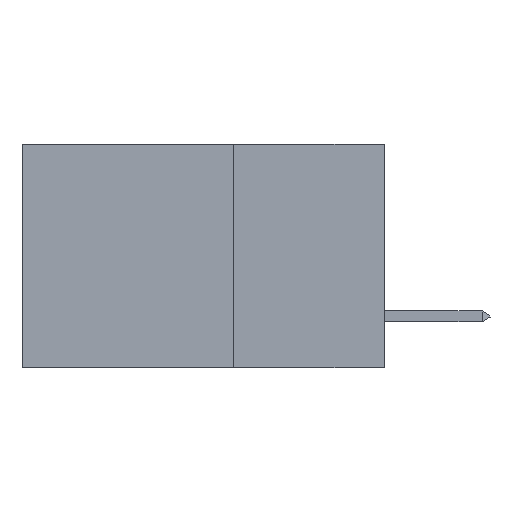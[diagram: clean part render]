
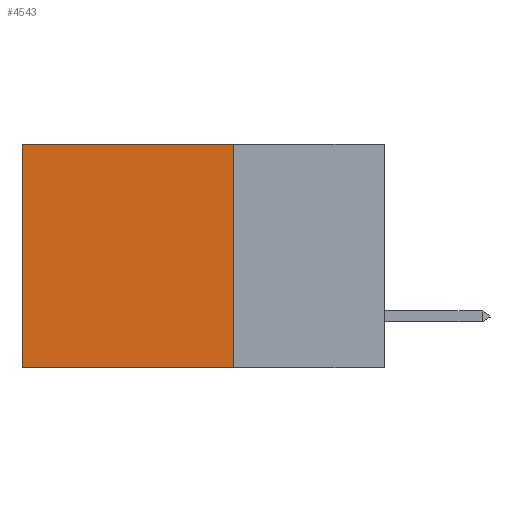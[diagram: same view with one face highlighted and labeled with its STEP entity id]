
A CAD part, left-side view. The second image highlights one B-rep face of the part: STEP entity #4543.
In plain terms, the highlighted planar face has unit normal (-1, 0, 0).
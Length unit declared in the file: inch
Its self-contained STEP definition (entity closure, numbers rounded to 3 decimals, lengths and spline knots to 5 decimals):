
#263 = ORIENTED_EDGE ( 'NONE', *, *, #15039, .F. ) ;
#498 = VERTEX_POINT ( 'NONE', #20043 ) ;
#1618 = DIRECTION ( 'NONE',  ( 0., 0., -1. ) ) ;
#2664 = CARTESIAN_POINT ( 'NONE',  ( 0.2875, 0.25, -0.37 ) ) ;
#3629 = CARTESIAN_POINT ( 'NONE',  ( 0.2875, 0.25, 0. ) ) ;
#3677 = VECTOR ( 'NONE', #28586, 39.37008 ) ;
#4152 = CARTESIAN_POINT ( 'NONE',  ( 0.2875, 0.25, 0. ) ) ;
#4487 = VERTEX_POINT ( 'NONE', #12778 ) ;
#4543 = ADVANCED_FACE ( 'NONE', ( #25303 ), #8254, .F. ) ;
#5996 = DIRECTION ( 'NONE',  ( 0., 0., -1. ) ) ;
#6521 = ORIENTED_EDGE ( 'NONE', *, *, #6524, .T. ) ;
#6524 = EDGE_CURVE ( 'NONE', #4487, #498, #29974, .T. ) ;
#8254 = PLANE ( 'NONE',  #13791 ) ;
#10584 = LINE ( 'NONE', #25099, #15299 ) ;
#12778 = CARTESIAN_POINT ( 'NONE',  ( 0.2875, 0.25, 0. ) ) ;
#13791 = AXIS2_PLACEMENT_3D ( 'NONE', #3629, #20010, #5996 ) ;
#14105 = ORIENTED_EDGE ( 'NONE', *, *, #14818, .F. ) ;
#14818 = EDGE_CURVE ( 'NONE', #23275, #22403, #22399, .T. ) ;
#15039 = EDGE_CURVE ( 'NONE', #4487, #23275, #17630, .T. ) ;
#15299 = VECTOR ( 'NONE', #1618, 39.37008 ) ;
#16179 = CARTESIAN_POINT ( 'NONE',  ( 0.2875, 0.25, -0.37 ) ) ;
#16893 = VECTOR ( 'NONE', #24563, 39.37008 ) ;
#17630 = LINE ( 'NONE', #19766, #16893 ) ;
#19766 = CARTESIAN_POINT ( 'NONE',  ( 0.2875, 0.25, 0. ) ) ;
#20010 = DIRECTION ( 'NONE',  ( 1., 0., 0. ) ) ;
#20043 = CARTESIAN_POINT ( 'NONE',  ( 0.2875, 0.6, 0. ) ) ;
#22157 = ORIENTED_EDGE ( 'NONE', *, *, #23154, .T. ) ;
#22399 = LINE ( 'NONE', #2664, #3677 ) ;
#22403 = VERTEX_POINT ( 'NONE', #29640 ) ;
#22733 = EDGE_LOOP ( 'NONE', ( #22157, #14105, #263, #6521 ) ) ;
#23154 = EDGE_CURVE ( 'NONE', #498, #22403, #10584, .T. ) ;
#23275 = VERTEX_POINT ( 'NONE', #16179 ) ;
#24563 = DIRECTION ( 'NONE',  ( 0., 0., -1. ) ) ;
#25099 = CARTESIAN_POINT ( 'NONE',  ( 0.2875, 0.6, 0. ) ) ;
#25303 = FACE_OUTER_BOUND ( 'NONE', #22733, .T. ) ;
#27492 = DIRECTION ( 'NONE',  ( 0., 1., 0. ) ) ;
#28586 = DIRECTION ( 'NONE',  ( 0., 1., 0. ) ) ;
#29259 = VECTOR ( 'NONE', #27492, 39.37008 ) ;
#29640 = CARTESIAN_POINT ( 'NONE',  ( 0.2875, 0.6, -0.37 ) ) ;
#29974 = LINE ( 'NONE', #4152, #29259 ) ;
